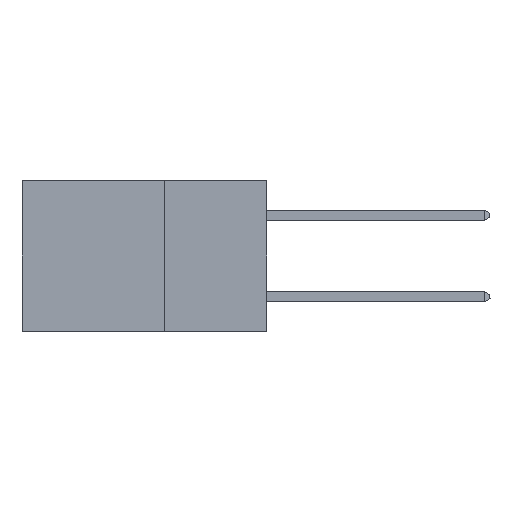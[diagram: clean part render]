
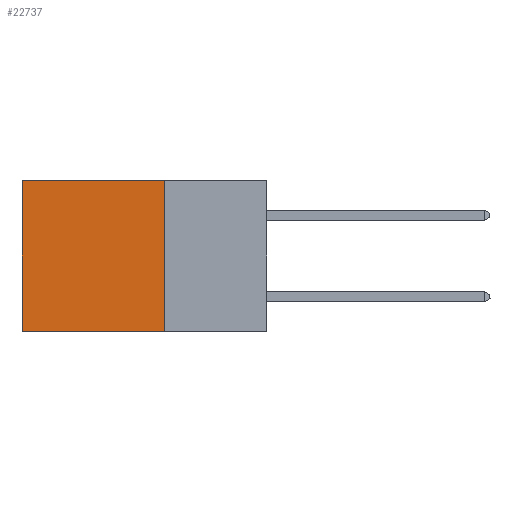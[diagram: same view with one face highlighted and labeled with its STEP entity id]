
A CAD part, left-side view. The second image highlights one B-rep face of the part: STEP entity #22737.
In plain terms, the highlighted planar face has unit normal (-1, 0, 0).
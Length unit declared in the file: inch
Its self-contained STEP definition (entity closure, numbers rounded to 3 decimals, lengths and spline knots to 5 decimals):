
#191 = VERTEX_POINT ( 'NONE', #15292 ) ;
#1546 = VECTOR ( 'NONE', #29847, 39.37008 ) ;
#1785 = EDGE_CURVE ( 'NONE', #10048, #10073, #12648, .T. ) ;
#2204 = CARTESIAN_POINT ( 'NONE',  ( 0.2875, 0.25, 0. ) ) ;
#3105 = VECTOR ( 'NONE', #13735, 39.37008 ) ;
#5367 = CARTESIAN_POINT ( 'NONE',  ( 0.2875, 0.6, -0.37 ) ) ;
#6358 = PLANE ( 'NONE',  #29345 ) ;
#7149 = EDGE_LOOP ( 'NONE', ( #10561, #8088, #8797, #28032 ) ) ;
#7978 = VERTEX_POINT ( 'NONE', #20979 ) ;
#8088 = ORIENTED_EDGE ( 'NONE', *, *, #1785, .F. ) ;
#8704 = DIRECTION ( 'NONE',  ( 0., 0., -1. ) ) ;
#8797 = ORIENTED_EDGE ( 'NONE', *, *, #9889, .F. ) ;
#9889 = EDGE_CURVE ( 'NONE', #7978, #10048, #18090, .T. ) ;
#10048 = VERTEX_POINT ( 'NONE', #10307 ) ;
#10073 = VERTEX_POINT ( 'NONE', #5367 ) ;
#10307 = CARTESIAN_POINT ( 'NONE',  ( 0.2875, 0.25, -0.37 ) ) ;
#10561 = ORIENTED_EDGE ( 'NONE', *, *, #26488, .T. ) ;
#12648 = LINE ( 'NONE', #14564, #16615 ) ;
#12863 = LINE ( 'NONE', #20870, #1546 ) ;
#13735 = DIRECTION ( 'NONE',  ( 0., 0., -1. ) ) ;
#14564 = CARTESIAN_POINT ( 'NONE',  ( 0.2875, 0.25, -0.37 ) ) ;
#14928 = CARTESIAN_POINT ( 'NONE',  ( 0.2875, 0.6, 0. ) ) ;
#15292 = CARTESIAN_POINT ( 'NONE',  ( 0.2875, 0.6, 0. ) ) ;
#16615 = VECTOR ( 'NONE', #17253, 39.37008 ) ;
#16912 = LINE ( 'NONE', #14928, #22495 ) ;
#17253 = DIRECTION ( 'NONE',  ( 0., 1., 0. ) ) ;
#18090 = LINE ( 'NONE', #2204, #3105 ) ;
#20109 = FACE_OUTER_BOUND ( 'NONE', #7149, .T. ) ;
#20301 = EDGE_CURVE ( 'NONE', #7978, #191, #12863, .T. ) ;
#20870 = CARTESIAN_POINT ( 'NONE',  ( 0.2875, 0.25, 0. ) ) ;
#20979 = CARTESIAN_POINT ( 'NONE',  ( 0.2875, 0.25, 0. ) ) ;
#22495 = VECTOR ( 'NONE', #29162, 39.37008 ) ;
#22728 = CARTESIAN_POINT ( 'NONE',  ( 0.2875, 0.25, 0. ) ) ;
#22737 = ADVANCED_FACE ( 'NONE', ( #20109 ), #6358, .F. ) ;
#26488 = EDGE_CURVE ( 'NONE', #191, #10073, #16912, .T. ) ;
#28032 = ORIENTED_EDGE ( 'NONE', *, *, #20301, .T. ) ;
#29162 = DIRECTION ( 'NONE',  ( 0., 0., -1. ) ) ;
#29345 = AXIS2_PLACEMENT_3D ( 'NONE', #22728, #29830, #8704 ) ;
#29830 = DIRECTION ( 'NONE',  ( 1., 0., 0. ) ) ;
#29847 = DIRECTION ( 'NONE',  ( 0., 1., 0. ) ) ;
